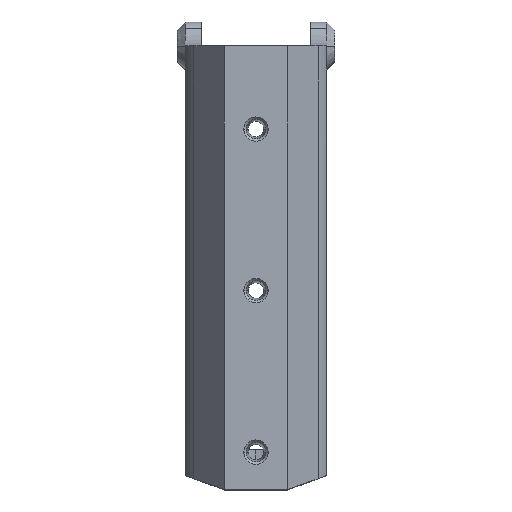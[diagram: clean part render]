
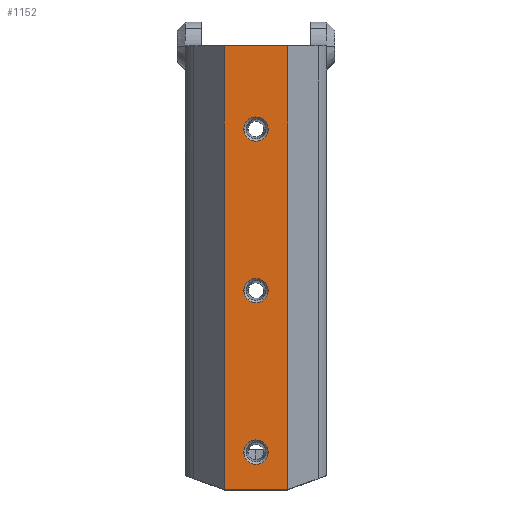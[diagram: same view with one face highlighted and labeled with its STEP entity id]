
A CAD part, top view. The second image highlights one B-rep face of the part: STEP entity #1152.
In plain terms, the highlighted face is planar.
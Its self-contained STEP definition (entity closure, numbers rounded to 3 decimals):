
#41 = VECTOR ( 'NONE', #6577, 1000. ) ;
#114 = DIRECTION ( 'NONE',  ( 0., 0., 1. ) ) ;
#125 = ORIENTED_EDGE ( 'NONE', *, *, #7176, .T. ) ;
#138 = VERTEX_POINT ( 'NONE', #5108 ) ;
#361 = EDGE_LOOP ( 'NONE', ( #4876, #1210 ) ) ;
#381 = CARTESIAN_POINT ( 'NONE',  ( 3., 41.311, -37.5 ) ) ;
#454 = VERTEX_POINT ( 'NONE', #3078 ) ;
#468 = DIRECTION ( 'NONE',  ( 0., 0., 1. ) ) ;
#469 = VERTEX_POINT ( 'NONE', #2001 ) ;
#476 = LINE ( 'NONE', #4488, #3057 ) ;
#650 = ORIENTED_EDGE ( 'NONE', *, *, #3536, .T. ) ;
#781 = FACE_BOUND ( 'NONE', #2514, .T. ) ;
#809 = CARTESIAN_POINT ( 'NONE',  ( -7.85, -165.097, -37.5 ) ) ;
#823 = CIRCLE ( 'NONE', #3002, 3. ) ;
#833 = ORIENTED_EDGE ( 'NONE', *, *, #4177, .F. ) ;
#869 = EDGE_CURVE ( 'NONE', #4789, #8046, #1703, .T. ) ;
#1001 = VERTEX_POINT ( 'NONE', #4744 ) ;
#1034 = DIRECTION ( 'NONE',  ( 0., 0., 1. ) ) ;
#1152 = ADVANCED_FACE ( 'NONE', ( #781, #2780, #4784, #2141 ), #8040, .F. ) ;
#1191 = AXIS2_PLACEMENT_3D ( 'NONE', #7527, #1034, #1717 ) ;
#1210 = ORIENTED_EDGE ( 'NONE', *, *, #869, .T. ) ;
#1222 = DIRECTION ( 'NONE',  ( -0.94, -0.342, 0. ) ) ;
#1267 = ORIENTED_EDGE ( 'NONE', *, *, #4842, .T. ) ;
#1332 = EDGE_CURVE ( 'NONE', #1416, #1001, #7869, .T. ) ;
#1370 = DIRECTION ( 'NONE',  ( 0., 0., 1. ) ) ;
#1386 = CARTESIAN_POINT ( 'NONE',  ( 7.832, 32.01, -37.5 ) ) ;
#1416 = VERTEX_POINT ( 'NONE', #3767 ) ;
#1703 = CIRCLE ( 'NONE', #2384, 3. ) ;
#1717 = DIRECTION ( 'NONE',  ( 1., 0., 0. ) ) ;
#2001 = CARTESIAN_POINT ( 'NONE',  ( 7.85, 141.911, -37.5 ) ) ;
#2041 = LINE ( 'NONE', #809, #5174 ) ;
#2137 = LINE ( 'NONE', #2736, #41 ) ;
#2141 = FACE_OUTER_BOUND ( 'NONE', #5139, .T. ) ;
#2316 = EDGE_CURVE ( 'NONE', #4118, #5530, #6204, .T. ) ;
#2384 = AXIS2_PLACEMENT_3D ( 'NONE', #3174, #6458, #2532 ) ;
#2514 = EDGE_LOOP ( 'NONE', ( #3417, #125 ) ) ;
#2532 = DIRECTION ( 'NONE',  ( 1., 0., 0. ) ) ;
#2602 = CARTESIAN_POINT ( 'NONE',  ( 0., 41.311, -37.5 ) ) ;
#2722 = CARTESIAN_POINT ( 'NONE',  ( 0., 121.311, -37.5 ) ) ;
#2733 = ORIENTED_EDGE ( 'NONE', *, *, #2316, .F. ) ;
#2736 = CARTESIAN_POINT ( 'NONE',  ( 7.85, -165.097, -37.5 ) ) ;
#2739 = CARTESIAN_POINT ( 'NONE',  ( 0., 81.311, -37.5 ) ) ;
#2748 = ORIENTED_EDGE ( 'NONE', *, *, #6985, .T. ) ;
#2780 = FACE_BOUND ( 'NONE', #4229, .T. ) ;
#2916 = EDGE_CURVE ( 'NONE', #6850, #469, #2137, .T. ) ;
#3002 = AXIS2_PLACEMENT_3D ( 'NONE', #2722, #114, #5326 ) ;
#3057 = VECTOR ( 'NONE', #3847, 1000. ) ;
#3078 = CARTESIAN_POINT ( 'NONE',  ( -3., 81.311, -37.5 ) ) ;
#3174 = CARTESIAN_POINT ( 'NONE',  ( 0., 41.311, -37.5 ) ) ;
#3329 = DIRECTION ( 'NONE',  ( 0., 0., 1. ) ) ;
#3417 = ORIENTED_EDGE ( 'NONE', *, *, #1332, .T. ) ;
#3536 = EDGE_CURVE ( 'NONE', #7708, #138, #2041, .T. ) ;
#3767 = CARTESIAN_POINT ( 'NONE',  ( -3., 121.311, -37.5 ) ) ;
#3798 = CARTESIAN_POINT ( 'NONE',  ( 0., 81.311, -37.5 ) ) ;
#3801 = AXIS2_PLACEMENT_3D ( 'NONE', #7395, #4150, #6754 ) ;
#3847 = DIRECTION ( 'NONE',  ( 0.94, -0.342, 0. ) ) ;
#4008 = CIRCLE ( 'NONE', #6334, 3. ) ;
#4118 = VERTEX_POINT ( 'NONE', #7300 ) ;
#4150 = DIRECTION ( 'NONE',  ( 0., 0., 1. ) ) ;
#4177 = EDGE_CURVE ( 'NONE', #469, #138, #6702, .T. ) ;
#4229 = EDGE_LOOP ( 'NONE', ( #1267, #6266 ) ) ;
#4269 = DIRECTION ( 'NONE',  ( -1., 0., 0. ) ) ;
#4435 = CARTESIAN_POINT ( 'NONE',  ( 3., 81.311, -37.5 ) ) ;
#4488 = CARTESIAN_POINT ( 'NONE',  ( 9.372, 25.748, -37.5 ) ) ;
#4509 = CARTESIAN_POINT ( 'NONE',  ( -9.372, 25.748, -37.5 ) ) ;
#4744 = CARTESIAN_POINT ( 'NONE',  ( 3., 121.311, -37.5 ) ) ;
#4784 = FACE_BOUND ( 'NONE', #361, .T. ) ;
#4789 = VERTEX_POINT ( 'NONE', #381 ) ;
#4842 = EDGE_CURVE ( 'NONE', #454, #8406, #6759, .T. ) ;
#4876 = ORIENTED_EDGE ( 'NONE', *, *, #5915, .T. ) ;
#5003 = CARTESIAN_POINT ( 'NONE',  ( 0., 32.01, -37.5 ) ) ;
#5108 = CARTESIAN_POINT ( 'NONE',  ( -7.85, 141.911, -37.5 ) ) ;
#5139 = EDGE_LOOP ( 'NONE', ( #5700, #650, #833, #7545, #2748, #2733 ) ) ;
#5174 = VECTOR ( 'NONE', #7942, 1000. ) ;
#5298 = VECTOR ( 'NONE', #6161, 1000. ) ;
#5326 = DIRECTION ( 'NONE',  ( 1., 0., 0. ) ) ;
#5530 = VERTEX_POINT ( 'NONE', #1386 ) ;
#5590 = DIRECTION ( 'NONE',  ( 1., 0., 0. ) ) ;
#5700 = ORIENTED_EDGE ( 'NONE', *, *, #6877, .F. ) ;
#5915 = EDGE_CURVE ( 'NONE', #8046, #4789, #8359, .T. ) ;
#6075 = AXIS2_PLACEMENT_3D ( 'NONE', #3798, #468, #5590 ) ;
#6161 = DIRECTION ( 'NONE',  ( 1., 0., 0. ) ) ;
#6204 = LINE ( 'NONE', #5003, #5298 ) ;
#6266 = ORIENTED_EDGE ( 'NONE', *, *, #6449, .T. ) ;
#6334 = AXIS2_PLACEMENT_3D ( 'NONE', #2739, #1370, #7353 ) ;
#6449 = EDGE_CURVE ( 'NONE', #8406, #454, #4008, .T. ) ;
#6458 = DIRECTION ( 'NONE',  ( 0., 0., 1. ) ) ;
#6577 = DIRECTION ( 'NONE',  ( 0., 1., 0. ) ) ;
#6662 = DIRECTION ( 'NONE',  ( 1., 0., 0. ) ) ;
#6702 = LINE ( 'NONE', #7384, #6900 ) ;
#6739 = CARTESIAN_POINT ( 'NONE',  ( -3., 41.311, -37.5 ) ) ;
#6754 = DIRECTION ( 'NONE',  ( 1., 0., 0. ) ) ;
#6759 = CIRCLE ( 'NONE', #6075, 3. ) ;
#6850 = VERTEX_POINT ( 'NONE', #7702 ) ;
#6877 = EDGE_CURVE ( 'NONE', #7708, #4118, #476, .T. ) ;
#6900 = VECTOR ( 'NONE', #4269, 1000. ) ;
#6985 = EDGE_CURVE ( 'NONE', #6850, #5530, #7763, .T. ) ;
#7176 = EDGE_CURVE ( 'NONE', #1001, #1416, #823, .T. ) ;
#7300 = CARTESIAN_POINT ( 'NONE',  ( -7.832, 32.01, -37.5 ) ) ;
#7353 = DIRECTION ( 'NONE',  ( 1., 0., 0. ) ) ;
#7365 = VECTOR ( 'NONE', #1222, 1000. ) ;
#7384 = CARTESIAN_POINT ( 'NONE',  ( 7.85, 141.911, -37.5 ) ) ;
#7395 = CARTESIAN_POINT ( 'NONE',  ( 0., -165.097, -37.5 ) ) ;
#7448 = CARTESIAN_POINT ( 'NONE',  ( -7.85, 32.016, -37.5 ) ) ;
#7527 = CARTESIAN_POINT ( 'NONE',  ( 0., 121.311, -37.5 ) ) ;
#7545 = ORIENTED_EDGE ( 'NONE', *, *, #2916, .F. ) ;
#7702 = CARTESIAN_POINT ( 'NONE',  ( 7.85, 32.016, -37.5 ) ) ;
#7708 = VERTEX_POINT ( 'NONE', #7448 ) ;
#7763 = LINE ( 'NONE', #4509, #7365 ) ;
#7869 = CIRCLE ( 'NONE', #1191, 3. ) ;
#7942 = DIRECTION ( 'NONE',  ( 0., 1., 0. ) ) ;
#8040 = PLANE ( 'NONE',  #3801 ) ;
#8046 = VERTEX_POINT ( 'NONE', #6739 ) ;
#8049 = AXIS2_PLACEMENT_3D ( 'NONE', #2602, #3329, #6662 ) ;
#8359 = CIRCLE ( 'NONE', #8049, 3. ) ;
#8406 = VERTEX_POINT ( 'NONE', #4435 ) ;
